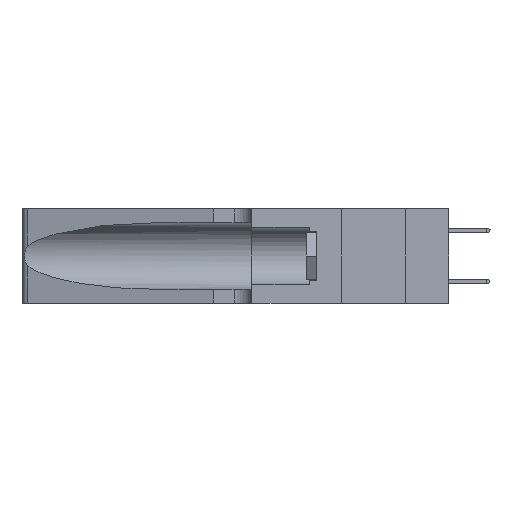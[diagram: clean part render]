
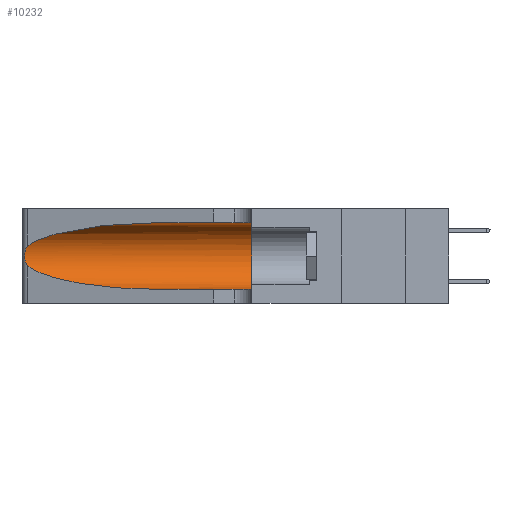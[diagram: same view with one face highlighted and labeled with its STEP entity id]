
A CAD part, left-side view. The second image highlights one B-rep face of the part: STEP entity #10232.
In plain terms, the highlighted cylindrical face has radius 3.308 mm (diameter 6.617 mm), a partial arc.
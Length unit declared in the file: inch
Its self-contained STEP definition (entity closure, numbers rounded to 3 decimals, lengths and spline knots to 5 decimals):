
#378 = CARTESIAN_POINT ( 'NONE',  ( 0.1305, 0.35, 0.31525 ) ) ;
#1418 = CARTESIAN_POINT ( 'NONE',  ( 0.1305, 0.35, 0.05475 ) ) ;
#1440 = EDGE_CURVE ( 'NONE', #14763, #24036, #13118, .T. ) ;
#1605 = DIRECTION ( 'NONE',  ( 0., 0., -1. ) ) ;
#1993 = CARTESIAN_POINT ( 'NONE',  ( 0.1305, 0.72297, 0.31525 ) ) ;
#2101 = CARTESIAN_POINT ( 'NONE',  ( 0.25639, 1.23186, 0.15144 ) ) ;
#2774 = EDGE_CURVE ( 'NONE', #32018, #14478, #5252, .T. ) ;
#3095 = DIRECTION ( 'NONE',  ( 0., -1., 0. ) ) ;
#3106 = B_SPLINE_CURVE_WITH_KNOTS ( 'NONE', 3,
 ( #4726, #19072, #7544, #30338, #12922, #30097, #35880, #4957, #16235, #35998, #4483, #2101, #24662, #15994 ),
 .UNSPECIFIED., .F., .F.,
 ( 4, 2, 2, 2, 2, 2, 4 ),
 ( 0., 0.00027, 0.00053, 0.00107, 0.0016, 0.00187, 0.00214 ),
 .UNSPECIFIED. ) ;
#4030 = LINE ( 'NONE', #12369, #15134 ) ;
#4483 = CARTESIAN_POINT ( 'NONE',  ( 0.25789, 1.23486, 0.15765 ) ) ;
#4726 = CARTESIAN_POINT ( 'NONE',  ( 0.25487, 1.22718, 0.22369 ) ) ;
#4957 = CARTESIAN_POINT ( 'NONE',  ( 0.26075, 1.23896, 0.178 ) ) ;
#5252 = CIRCLE ( 'NONE', #33363, 0.13025 ) ;
#5816 = EDGE_CURVE ( 'NONE', #24036, #9486, #3106, .T. ) ;
#6783 = ORIENTED_EDGE ( 'NONE', *, *, #1440, .T. ) ;
#6841 = VECTOR ( 'NONE', #3095, 39.37008 ) ;
#7011 = ORIENTED_EDGE ( 'NONE', *, *, #5816, .T. ) ;
#7291 = CARTESIAN_POINT ( 'NONE',  ( 0.18966, 0.96281, 0.05475 ) ) ;
#7544 = CARTESIAN_POINT ( 'NONE',  ( 0.25639, 1.23184, 0.21858 ) ) ;
#8079 =( BOUNDED_CURVE ( )  B_SPLINE_CURVE ( 3, ( #23938, #24300, #7291, #18589 ),
 .UNSPECIFIED., .F., .F. ) 
 B_SPLINE_CURVE_WITH_KNOTS ( ( 4, 4 ),
 ( 3.44316, 4.71239 ),
 .UNSPECIFIED. ) 
 CURVE ( )  GEOMETRIC_REPRESENTATION_ITEM ( )  RATIONAL_B_SPLINE_CURVE ( ( 1., 0.87, 0.87, 1. ) ) 
 REPRESENTATION_ITEM ( '' )  );
#9278 = ORIENTED_EDGE ( 'NONE', *, *, #2774, .F. ) ;
#9374 = CARTESIAN_POINT ( 'NONE',  ( 0.25487, 1.22718, 0.22369 ) ) ;
#9486 = VERTEX_POINT ( 'NONE', #9561 ) ;
#9561 = CARTESIAN_POINT ( 'NONE',  ( 0.25487, 1.22718, 0.14631 ) ) ;
#9772 = EDGE_CURVE ( 'NONE', #14763, #32018, #12174, .T. ) ;
#10232 = ADVANCED_FACE ( 'NONE', ( #13441 ), #16098, .F. ) ;
#11362 = DIRECTION ( 'NONE',  ( 0., -1., 0. ) ) ;
#12174 = LINE ( 'NONE', #14511, #6841 ) ;
#12369 = CARTESIAN_POINT ( 'NONE',  ( 0.1305, 1.61858, 0.05475 ) ) ;
#12922 = CARTESIAN_POINT ( 'NONE',  ( 0.25854, 1.2359, 0.20912 ) ) ;
#13118 =( BOUNDED_CURVE ( )  B_SPLINE_CURVE ( 3, ( #1993, #32950, #24666, #29858 ),
 .UNSPECIFIED., .F., .F. ) 
 B_SPLINE_CURVE_WITH_KNOTS ( ( 4, 4 ),
 ( 1.5708, 2.84003 ),
 .UNSPECIFIED. ) 
 CURVE ( )  GEOMETRIC_REPRESENTATION_ITEM ( )  RATIONAL_B_SPLINE_CURVE ( ( 1., 0.87, 0.87, 1. ) ) 
 REPRESENTATION_ITEM ( '' )  );
#13441 = FACE_OUTER_BOUND ( 'NONE', #21022, .T. ) ;
#14369 = CARTESIAN_POINT ( 'NONE',  ( 0.1305, 0.72297, 0.05475 ) ) ;
#14478 = VERTEX_POINT ( 'NONE', #1418 ) ;
#14511 = CARTESIAN_POINT ( 'NONE',  ( 0.1305, 1.61858, 0.31525 ) ) ;
#14763 = VERTEX_POINT ( 'NONE', #25302 ) ;
#14806 = DIRECTION ( 'NONE',  ( 0., 1., 0. ) ) ;
#15134 = VECTOR ( 'NONE', #11362, 39.37008 ) ;
#15418 = ORIENTED_EDGE ( 'NONE', *, *, #21688, .T. ) ;
#15994 = CARTESIAN_POINT ( 'NONE',  ( 0.25487, 1.22718, 0.14631 ) ) ;
#16098 = CYLINDRICAL_SURFACE ( 'NONE', #33520, 0.13025 ) ;
#16235 = CARTESIAN_POINT ( 'NONE',  ( 0.26017, 1.23833, 0.17102 ) ) ;
#18589 = CARTESIAN_POINT ( 'NONE',  ( 0.1305, 0.72297, 0.05475 ) ) ;
#18857 = EDGE_CURVE ( 'NONE', #22070, #14478, #4030, .T. ) ;
#19072 = CARTESIAN_POINT ( 'NONE',  ( 0.25555, 1.22994, 0.2215 ) ) ;
#20513 = ORIENTED_EDGE ( 'NONE', *, *, #9772, .F. ) ;
#21022 = EDGE_LOOP ( 'NONE', ( #6783, #7011, #15418, #36321, #9278, #20513 ) ) ;
#21653 = DIRECTION ( 'NONE',  ( 0., -1., 0. ) ) ;
#21688 = EDGE_CURVE ( 'NONE', #9486, #22070, #8079, .T. ) ;
#22070 = VERTEX_POINT ( 'NONE', #14369 ) ;
#22872 = CARTESIAN_POINT ( 'NONE',  ( 0.1305, 0.35, 0.185 ) ) ;
#23938 = CARTESIAN_POINT ( 'NONE',  ( 0.25487, 1.22718, 0.14631 ) ) ;
#24036 = VERTEX_POINT ( 'NONE', #9374 ) ;
#24300 = CARTESIAN_POINT ( 'NONE',  ( 0.2373, 1.15595, 0.08982 ) ) ;
#24662 = CARTESIAN_POINT ( 'NONE',  ( 0.25555, 1.22993, 0.14849 ) ) ;
#24666 = CARTESIAN_POINT ( 'NONE',  ( 0.2373, 1.15595, 0.28018 ) ) ;
#25302 = CARTESIAN_POINT ( 'NONE',  ( 0.1305, 0.72297, 0.31525 ) ) ;
#25828 = DIRECTION ( 'NONE',  ( 0., 0., 1. ) ) ;
#29858 = CARTESIAN_POINT ( 'NONE',  ( 0.25487, 1.22718, 0.22369 ) ) ;
#30097 = CARTESIAN_POINT ( 'NONE',  ( 0.26018, 1.23835, 0.19895 ) ) ;
#30338 = CARTESIAN_POINT ( 'NONE',  ( 0.25787, 1.23484, 0.2124 ) ) ;
#32018 = VERTEX_POINT ( 'NONE', #378 ) ;
#32950 = CARTESIAN_POINT ( 'NONE',  ( 0.18966, 0.96281, 0.31525 ) ) ;
#33256 = CARTESIAN_POINT ( 'NONE',  ( 0.1305, 1.61858, 0.185 ) ) ;
#33363 = AXIS2_PLACEMENT_3D ( 'NONE', #22872, #14806, #25828 ) ;
#33520 = AXIS2_PLACEMENT_3D ( 'NONE', #33256, #21653, #1605 ) ;
#35880 = CARTESIAN_POINT ( 'NONE',  ( 0.26075, 1.23896, 0.19203 ) ) ;
#35998 = CARTESIAN_POINT ( 'NONE',  ( 0.25856, 1.23593, 0.16098 ) ) ;
#36321 = ORIENTED_EDGE ( 'NONE', *, *, #18857, .T. ) ;
